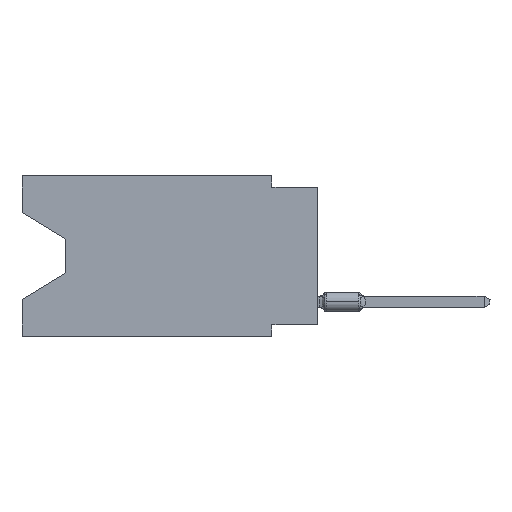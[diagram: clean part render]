
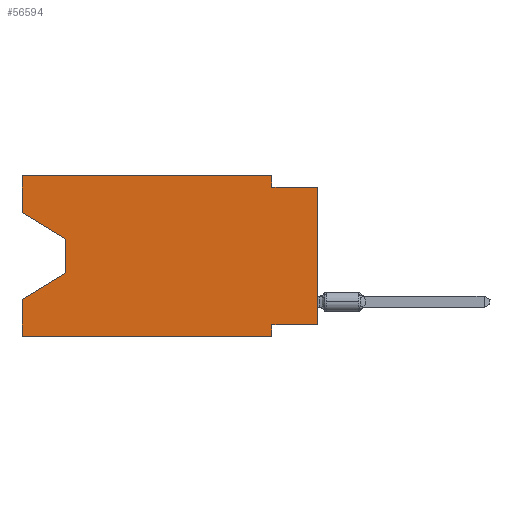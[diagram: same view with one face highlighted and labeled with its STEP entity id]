
A CAD part, left-side view. The second image highlights one B-rep face of the part: STEP entity #56594.
In plain terms, the highlighted planar face has unit normal (-1, 0, 0).
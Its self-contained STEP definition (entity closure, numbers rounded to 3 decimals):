
#1020 = CARTESIAN_POINT ( 'NONE',  ( 0., 13.97, -5.385 ) ) ;
#3228 = VERTEX_POINT ( 'NONE', #29337 ) ;
#4052 = EDGE_CURVE ( 'NONE', #57969, #7416, #18828, .T. ) ;
#4869 = CARTESIAN_POINT ( 'NONE',  ( 0., 2.54, -0.635 ) ) ;
#4926 = ORIENTED_EDGE ( 'NONE', *, *, #54250, .F. ) ;
#6154 = EDGE_LOOP ( 'NONE', ( #47851, #35832, #46680, #56654, #22714, #64709, #37586, #51351, #39640, #44928, #4926, #36629 ) ) ;
#6317 = LINE ( 'NONE', #28618, #22304 ) ;
#7416 = VERTEX_POINT ( 'NONE', #25009 ) ;
#7545 = VERTEX_POINT ( 'NONE', #38148 ) ;
#9469 = VECTOR ( 'NONE', #23745, 1000. ) ;
#10138 = LINE ( 'NONE', #60302, #45788 ) ;
#10623 = EDGE_CURVE ( 'NONE', #64516, #28849, #6317, .T. ) ;
#12613 = VECTOR ( 'NONE', #66601, 1000. ) ;
#14897 = CARTESIAN_POINT ( 'NONE',  ( 0., 16.383, 0. ) ) ;
#14950 = VERTEX_POINT ( 'NONE', #18985 ) ;
#15363 = VECTOR ( 'NONE', #38852, 1000. ) ;
#16847 = VECTOR ( 'NONE', #65084, 1000. ) ;
#17346 = EDGE_CURVE ( 'NONE', #64516, #57969, #22863, .T. ) ;
#18828 = LINE ( 'NONE', #46306, #47132 ) ;
#18985 = CARTESIAN_POINT ( 'NONE',  ( 0., 2.54, 0. ) ) ;
#20219 = CARTESIAN_POINT ( 'NONE',  ( 0., 0., -8.255 ) ) ;
#20447 = EDGE_CURVE ( 'NONE', #30881, #3228, #50523, .T. ) ;
#21688 = VECTOR ( 'NONE', #57285, 1000. ) ;
#22304 = VECTOR ( 'NONE', #50239, 1000. ) ;
#22697 = EDGE_CURVE ( 'NONE', #7416, #3228, #28805, .T. ) ;
#22714 = ORIENTED_EDGE ( 'NONE', *, *, #31343, .T. ) ;
#22863 = LINE ( 'NONE', #33854, #63850 ) ;
#23392 = CARTESIAN_POINT ( 'NONE',  ( 0., 16.383, 0. ) ) ;
#23745 = DIRECTION ( 'NONE',  ( 0., 0., -1. ) ) ;
#25007 = CARTESIAN_POINT ( 'NONE',  ( 0., 2.54, -8.89 ) ) ;
#25009 = CARTESIAN_POINT ( 'NONE',  ( 0., 13.97, -5.385 ) ) ;
#25062 = FACE_OUTER_BOUND ( 'NONE', #6154, .T. ) ;
#25064 = EDGE_CURVE ( 'NONE', #7545, #34964, #71380, .T. ) ;
#25610 = CARTESIAN_POINT ( 'NONE',  ( 0., 16.383, 0. ) ) ;
#26110 = VECTOR ( 'NONE', #62965, 1000. ) ;
#26448 = EDGE_CURVE ( 'NONE', #39078, #68052, #45814, .T. ) ;
#28618 = CARTESIAN_POINT ( 'NONE',  ( 0., 16.383, 0. ) ) ;
#28805 = LINE ( 'NONE', #1020, #49940 ) ;
#28849 = VERTEX_POINT ( 'NONE', #25610 ) ;
#29337 = CARTESIAN_POINT ( 'NONE',  ( 0., 16.383, -6.852 ) ) ;
#30345 = EDGE_CURVE ( 'NONE', #39078, #7545, #66696, .T. ) ;
#30881 = VERTEX_POINT ( 'NONE', #36117 ) ;
#31343 = EDGE_CURVE ( 'NONE', #30881, #34964, #64229, .T. ) ;
#33854 = CARTESIAN_POINT ( 'NONE',  ( 0., 16.383, -2.038 ) ) ;
#34964 = VERTEX_POINT ( 'NONE', #25007 ) ;
#35468 = CARTESIAN_POINT ( 'NONE',  ( 0., 2.54, 0. ) ) ;
#35832 = ORIENTED_EDGE ( 'NONE', *, *, #4052, .T. ) ;
#36117 = CARTESIAN_POINT ( 'NONE',  ( 0., 16.383, -8.89 ) ) ;
#36629 = ORIENTED_EDGE ( 'NONE', *, *, #10623, .F. ) ;
#37586 = ORIENTED_EDGE ( 'NONE', *, *, #30345, .F. ) ;
#38148 = CARTESIAN_POINT ( 'NONE',  ( 0., 2.54, -8.255 ) ) ;
#38852 = DIRECTION ( 'NONE',  ( 0., 1., 0. ) ) ;
#39078 = VERTEX_POINT ( 'NONE', #20219 ) ;
#39640 = ORIENTED_EDGE ( 'NONE', *, *, #50197, .F. ) ;
#39749 = EDGE_CURVE ( 'NONE', #14950, #61501, #68435, .T. ) ;
#39802 = DIRECTION ( 'NONE',  ( 0., 0.855, -0.519 ) ) ;
#44252 = CARTESIAN_POINT ( 'NONE',  ( 0., 2.54, -8.89 ) ) ;
#44928 = ORIENTED_EDGE ( 'NONE', *, *, #39749, .F. ) ;
#45788 = VECTOR ( 'NONE', #72355, 1000. ) ;
#45814 = LINE ( 'NONE', #50217, #50190 ) ;
#46306 = CARTESIAN_POINT ( 'NONE',  ( 0., 13.97, -3.505 ) ) ;
#46680 = ORIENTED_EDGE ( 'NONE', *, *, #22697, .T. ) ;
#47132 = VECTOR ( 'NONE', #57675, 1000. ) ;
#47851 = ORIENTED_EDGE ( 'NONE', *, *, #17346, .T. ) ;
#48230 = LINE ( 'NONE', #14897, #16847 ) ;
#49940 = VECTOR ( 'NONE', #39802, 1000. ) ;
#50190 = VECTOR ( 'NONE', #61203, 1000. ) ;
#50197 = EDGE_CURVE ( 'NONE', #61501, #68052, #10138, .T. ) ;
#50217 = CARTESIAN_POINT ( 'NONE',  ( 0., 0., 0. ) ) ;
#50239 = DIRECTION ( 'NONE',  ( 0., 0., 1. ) ) ;
#50523 = LINE ( 'NONE', #23392, #26110 ) ;
#50588 = CARTESIAN_POINT ( 'NONE',  ( 0., 0., -8.255 ) ) ;
#50619 = CARTESIAN_POINT ( 'NONE',  ( 0., 0., -0.635 ) ) ;
#51351 = ORIENTED_EDGE ( 'NONE', *, *, #26448, .T. ) ;
#51531 = DIRECTION ( 'NONE',  ( 0., 0., -1. ) ) ;
#53011 = CARTESIAN_POINT ( 'NONE',  ( 0., 13.97, -3.505 ) ) ;
#54250 = EDGE_CURVE ( 'NONE', #28849, #14950, #48230, .T. ) ;
#56211 = DIRECTION ( 'NONE',  ( 0., -0.855, -0.519 ) ) ;
#56594 = ADVANCED_FACE ( 'NONE', ( #25062 ), #62531, .F. ) ;
#56654 = ORIENTED_EDGE ( 'NONE', *, *, #20447, .F. ) ;
#56683 = CARTESIAN_POINT ( 'NONE',  ( 0., 16.383, 0. ) ) ;
#57285 = DIRECTION ( 'NONE',  ( 0., -1., 0. ) ) ;
#57675 = DIRECTION ( 'NONE',  ( 0., 0., -1. ) ) ;
#57969 = VERTEX_POINT ( 'NONE', #53011 ) ;
#58775 = DIRECTION ( 'NONE',  ( 1., 0., 0. ) ) ;
#60302 = CARTESIAN_POINT ( 'NONE',  ( 0., 0., -0.635 ) ) ;
#61203 = DIRECTION ( 'NONE',  ( 0., 0., 1. ) ) ;
#61501 = VERTEX_POINT ( 'NONE', #4869 ) ;
#62531 = PLANE ( 'NONE',  #64191 ) ;
#62965 = DIRECTION ( 'NONE',  ( 0., 0., 1. ) ) ;
#63850 = VECTOR ( 'NONE', #56211, 1000. ) ;
#64191 = AXIS2_PLACEMENT_3D ( 'NONE', #56683, #58775, #51531 ) ;
#64229 = LINE ( 'NONE', #69717, #21688 ) ;
#64516 = VERTEX_POINT ( 'NONE', #69540 ) ;
#64709 = ORIENTED_EDGE ( 'NONE', *, *, #25064, .F. ) ;
#65084 = DIRECTION ( 'NONE',  ( 0., -1., 0. ) ) ;
#66601 = DIRECTION ( 'NONE',  ( 0., 0., -1. ) ) ;
#66696 = LINE ( 'NONE', #50588, #15363 ) ;
#68052 = VERTEX_POINT ( 'NONE', #50619 ) ;
#68435 = LINE ( 'NONE', #35468, #9469 ) ;
#69540 = CARTESIAN_POINT ( 'NONE',  ( 0., 16.383, -2.038 ) ) ;
#69717 = CARTESIAN_POINT ( 'NONE',  ( 0., 16.383, -8.89 ) ) ;
#71380 = LINE ( 'NONE', #44252, #12613 ) ;
#72355 = DIRECTION ( 'NONE',  ( 0., -1., 0. ) ) ;
